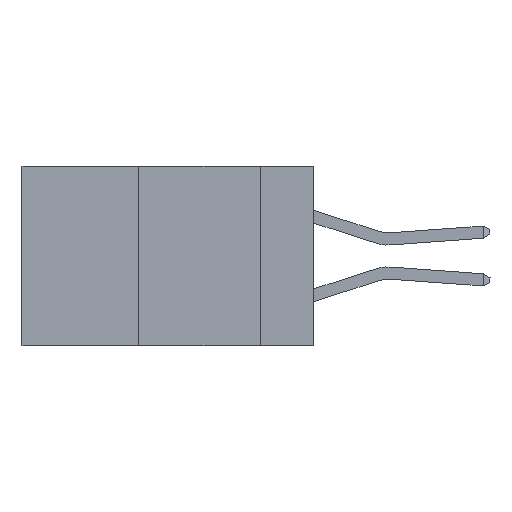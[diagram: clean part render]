
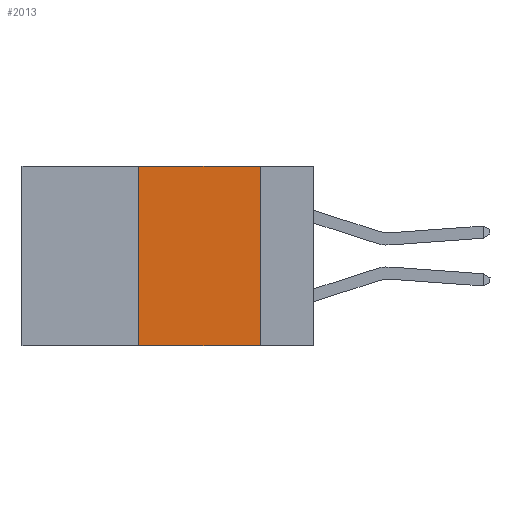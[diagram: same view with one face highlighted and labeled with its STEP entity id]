
A CAD part, left-side view. The second image highlights one B-rep face of the part: STEP entity #2013.
In plain terms, the highlighted planar face has unit normal (-1, 0, 0).
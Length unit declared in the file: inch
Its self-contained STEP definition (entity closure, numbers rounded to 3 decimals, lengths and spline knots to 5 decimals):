
#740 = DIRECTION ( 'NONE',  ( 1., 0., 0. ) ) ;
#1045 = VERTEX_POINT ( 'NONE', #6567 ) ;
#2013 = ADVANCED_FACE ( 'NONE', ( #27503 ), #5335, .F. ) ;
#2433 = VECTOR ( 'NONE', #22652, 39.37008 ) ;
#2931 = EDGE_CURVE ( 'NONE', #7500, #1045, #10469, .T. ) ;
#4494 = CARTESIAN_POINT ( 'NONE',  ( 0., 0.36, -0.37 ) ) ;
#5335 = PLANE ( 'NONE',  #5686 ) ;
#5686 = AXIS2_PLACEMENT_3D ( 'NONE', #14701, #740, #17066 ) ;
#6346 = CARTESIAN_POINT ( 'NONE',  ( 0., 0.11, 0. ) ) ;
#6567 = CARTESIAN_POINT ( 'NONE',  ( 0., 0.36, 0. ) ) ;
#6631 = EDGE_LOOP ( 'NONE', ( #26916, #8902, #8556, #6799 ) ) ;
#6799 = ORIENTED_EDGE ( 'NONE', *, *, #12817, .T. ) ;
#7500 = VERTEX_POINT ( 'NONE', #4494 ) ;
#8556 = ORIENTED_EDGE ( 'NONE', *, *, #2931, .F. ) ;
#8902 = ORIENTED_EDGE ( 'NONE', *, *, #9317, .F. ) ;
#9317 = EDGE_CURVE ( 'NONE', #1045, #22968, #29289, .T. ) ;
#10469 = LINE ( 'NONE', #20594, #14532 ) ;
#10827 = CARTESIAN_POINT ( 'NONE',  ( 0., 0.11, -0.37 ) ) ;
#10932 = VECTOR ( 'NONE', #20413, 39.37008 ) ;
#12004 = DIRECTION ( 'NONE',  ( 0., -1., 0. ) ) ;
#12817 = EDGE_CURVE ( 'NONE', #7500, #20741, #21153, .T. ) ;
#14501 = CARTESIAN_POINT ( 'NONE',  ( 0., 0.11, 0. ) ) ;
#14532 = VECTOR ( 'NONE', #27387, 39.37008 ) ;
#14701 = CARTESIAN_POINT ( 'NONE',  ( 0., 0.6, 0. ) ) ;
#14939 = VECTOR ( 'NONE', #12004, 39.37008 ) ;
#17066 = DIRECTION ( 'NONE',  ( 0., 0., -1. ) ) ;
#19058 = CARTESIAN_POINT ( 'NONE',  ( 0., 0.6, -0.37 ) ) ;
#20086 = EDGE_CURVE ( 'NONE', #22968, #20741, #20327, .T. ) ;
#20327 = LINE ( 'NONE', #6346, #2433 ) ;
#20413 = DIRECTION ( 'NONE',  ( 0., -1., 0. ) ) ;
#20594 = CARTESIAN_POINT ( 'NONE',  ( 0., 0.36, 0. ) ) ;
#20741 = VERTEX_POINT ( 'NONE', #10827 ) ;
#21153 = LINE ( 'NONE', #19058, #14939 ) ;
#22652 = DIRECTION ( 'NONE',  ( 0., 0., -1. ) ) ;
#22968 = VERTEX_POINT ( 'NONE', #14501 ) ;
#24961 = CARTESIAN_POINT ( 'NONE',  ( 0., 0.6, 0. ) ) ;
#26916 = ORIENTED_EDGE ( 'NONE', *, *, #20086, .F. ) ;
#27387 = DIRECTION ( 'NONE',  ( 0., 0., 1. ) ) ;
#27503 = FACE_OUTER_BOUND ( 'NONE', #6631, .T. ) ;
#29289 = LINE ( 'NONE', #24961, #10932 ) ;
